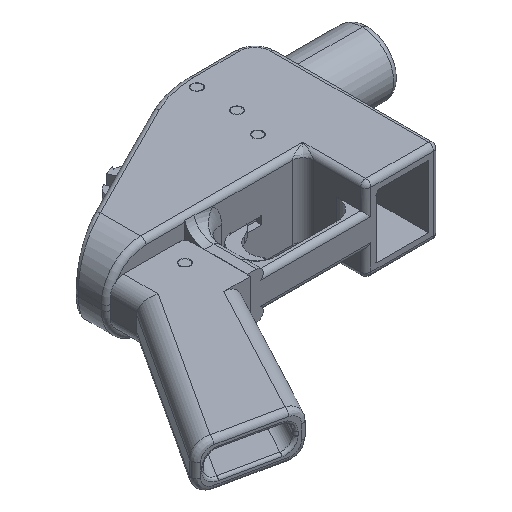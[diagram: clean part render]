
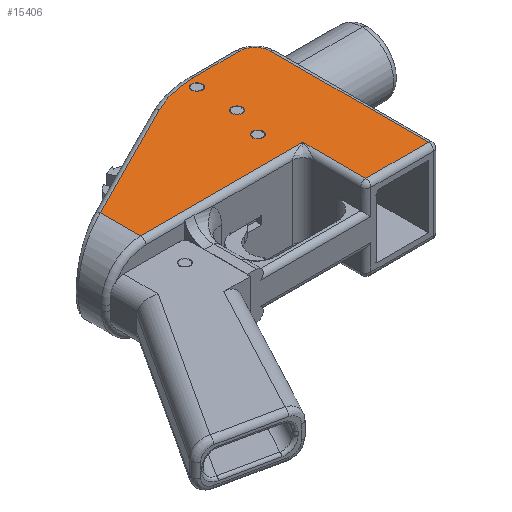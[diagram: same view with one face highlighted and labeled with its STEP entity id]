
A CAD part, isometric view. The second image highlights one B-rep face of the part: STEP entity #15406.
In plain terms, the highlighted planar face has unit normal (0, 0, 1).
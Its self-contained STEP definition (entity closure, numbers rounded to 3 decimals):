
#90 = EDGE_CURVE ( 'NONE', #6622, #9751, #9383, .T. ) ;
#178 = EDGE_CURVE ( 'NONE', #16074, #3045, #4969, .T. ) ;
#243 = VECTOR ( 'NONE', #9661, 1000. ) ;
#358 = DIRECTION ( 'NONE',  ( -0.893, -0.45, 0. ) ) ;
#572 = DIRECTION ( 'NONE',  ( 1., 0., 0. ) ) ;
#606 = DIRECTION ( 'NONE',  ( 1., 0., 0. ) ) ;
#698 = CARTESIAN_POINT ( 'NONE',  ( -33.02, 0., 40.64 ) ) ;
#745 = AXIS2_PLACEMENT_3D ( 'NONE', #16771, #8692, #606 ) ;
#792 = CARTESIAN_POINT ( 'NONE',  ( -32.373, 8.026, 40.64 ) ) ;
#1015 = ORIENTED_EDGE ( 'NONE', *, *, #2822, .F. ) ;
#1487 = PLANE ( 'NONE',  #14224 ) ;
#1628 = CARTESIAN_POINT ( 'NONE',  ( -10.16, 48.666, 40.64 ) ) ;
#1798 = VERTEX_POINT ( 'NONE', #6465 ) ;
#1871 = AXIS2_PLACEMENT_3D ( 'NONE', #6925, #16336, #8287 ) ;
#1890 = FACE_BOUND ( 'NONE', #12005, .T. ) ;
#2166 = DIRECTION ( 'NONE',  ( 1., 0., 0. ) ) ;
#2328 = ORIENTED_EDGE ( 'NONE', *, *, #14817, .T. ) ;
#2641 = EDGE_CURVE ( 'NONE', #2721, #5325, #10907, .T. ) ;
#2650 = CARTESIAN_POINT ( 'NONE',  ( -111.887, 21.996, 40.64 ) ) ;
#2721 = VERTEX_POINT ( 'NONE', #2773 ) ;
#2773 = CARTESIAN_POINT ( 'NONE',  ( -33.02, 32.004, 40.64 ) ) ;
#2795 = ORIENTED_EDGE ( 'NONE', *, *, #5868, .T. ) ;
#2805 = CARTESIAN_POINT ( 'NONE',  ( -32.373, 56.286, 40.64 ) ) ;
#2822 = EDGE_CURVE ( 'NONE', #15205, #1798, #7974, .T. ) ;
#2852 = DIRECTION ( 'NONE',  ( 0., 0., 1. ) ) ;
#2897 = CARTESIAN_POINT ( 'NONE',  ( -33.02, -27.94, 40.64 ) ) ;
#2994 = DIRECTION ( 'NONE',  ( 1., 0., 0. ) ) ;
#3013 = ORIENTED_EDGE ( 'NONE', *, *, #15553, .T. ) ;
#3045 = VERTEX_POINT ( 'NONE', #10293 ) ;
#3214 = ORIENTED_EDGE ( 'NONE', *, *, #6629, .T. ) ;
#3539 = DIRECTION ( 'NONE',  ( 1., 0., 0. ) ) ;
#3587 = CARTESIAN_POINT ( 'NONE',  ( -2.54, -27.94, 40.64 ) ) ;
#3727 = CARTESIAN_POINT ( 'NONE',  ( -35.56, 32.004, 40.64 ) ) ;
#4057 = VECTOR ( 'NONE', #12836, 1000. ) ;
#4969 = LINE ( 'NONE', #8660, #8136 ) ;
#5080 = DIRECTION ( 'NONE',  ( 1., 0., 0. ) ) ;
#5325 = VERTEX_POINT ( 'NONE', #15192 ) ;
#5681 = CARTESIAN_POINT ( 'NONE',  ( -35.56, 51.46, 40.64 ) ) ;
#5856 = VERTEX_POINT ( 'NONE', #2897 ) ;
#5868 = EDGE_CURVE ( 'NONE', #12746, #16471, #7442, .T. ) ;
#6081 = EDGE_CURVE ( 'NONE', #7611, #16074, #7645, .T. ) ;
#6192 = CARTESIAN_POINT ( 'NONE',  ( 0., -27.94, 40.64 ) ) ;
#6370 = ORIENTED_EDGE ( 'NONE', *, *, #14451, .T. ) ;
#6440 = EDGE_LOOP ( 'NONE', ( #9652, #13041, #6370, #2795, #2328, #6658, #3214, #3013, #10388 ) ) ;
#6465 = CARTESIAN_POINT ( 'NONE',  ( -33.02, 51.46, 40.64 ) ) ;
#6622 = VERTEX_POINT ( 'NONE', #11529 ) ;
#6629 = EDGE_CURVE ( 'NONE', #16402, #8328, #9920, .T. ) ;
#6658 = ORIENTED_EDGE ( 'NONE', *, *, #7137, .T. ) ;
#6925 = CARTESIAN_POINT ( 'NONE',  ( -40.64, 16.764, 40.64 ) ) ;
#7032 = ORIENTED_EDGE ( 'NONE', *, *, #90, .F. ) ;
#7036 = DIRECTION ( 'NONE',  ( 1., 0., 0. ) ) ;
#7069 = CARTESIAN_POINT ( 'NONE',  ( -35.56, 51.46, 40.64 ) ) ;
#7137 = EDGE_CURVE ( 'NONE', #11227, #16402, #10328, .T. ) ;
#7325 = EDGE_CURVE ( 'NONE', #3045, #5856, #8636, .T. ) ;
#7442 = LINE ( 'NONE', #8320, #243 ) ;
#7443 = DIRECTION ( 'NONE',  ( 0., -1., 0. ) ) ;
#7601 = CARTESIAN_POINT ( 'NONE',  ( -35.56, 32.004, 40.64 ) ) ;
#7611 = VERTEX_POINT ( 'NONE', #2650 ) ;
#7645 = LINE ( 'NONE', #10128, #4057 ) ;
#7696 = CARTESIAN_POINT ( 'NONE',  ( -38.1, 51.46, 40.64 ) ) ;
#7916 = EDGE_CURVE ( 'NONE', #5325, #2721, #10829, .T. ) ;
#7974 = CIRCLE ( 'NONE', #9037, 2.54 ) ;
#8136 = VECTOR ( 'NONE', #572, 1000. ) ;
#8287 = DIRECTION ( 'NONE',  ( 1., 0., 0. ) ) ;
#8320 = CARTESIAN_POINT ( 'NONE',  ( -2.54, 48.666, 40.64 ) ) ;
#8328 = VERTEX_POINT ( 'NONE', #11096 ) ;
#8422 = DIRECTION ( 'NONE',  ( 1., 0., 0. ) ) ;
#8543 = ORIENTED_EDGE ( 'NONE', *, *, #2641, .F. ) ;
#8633 = FACE_OUTER_BOUND ( 'NONE', #6440, .T. ) ;
#8636 = LINE ( 'NONE', #698, #11377 ) ;
#8660 = CARTESIAN_POINT ( 'NONE',  ( -35.56, 2.54, 40.64 ) ) ;
#8692 = DIRECTION ( 'NONE',  ( 0., 0., 1. ) ) ;
#8703 = CARTESIAN_POINT ( 'NONE',  ( -111.887, 2.54, 40.64 ) ) ;
#8934 = DIRECTION ( 'NONE',  ( 1., 0., 0. ) ) ;
#9037 = AXIS2_PLACEMENT_3D ( 'NONE', #7069, #16488, #8422 ) ;
#9312 = AXIS2_PLACEMENT_3D ( 'NONE', #5681, #15102, #7036 ) ;
#9366 = AXIS2_PLACEMENT_3D ( 'NONE', #792, #10224, #2166 ) ;
#9383 = CIRCLE ( 'NONE', #745, 2.54 ) ;
#9475 = FACE_BOUND ( 'NONE', #13864, .T. ) ;
#9652 = ORIENTED_EDGE ( 'NONE', *, *, #178, .T. ) ;
#9661 = DIRECTION ( 'NONE',  ( 0., 1., 0. ) ) ;
#9751 = VERTEX_POINT ( 'NONE', #15191 ) ;
#9780 = CARTESIAN_POINT ( 'NONE',  ( -110.744, 22.572, 40.64 ) ) ;
#9920 = CIRCLE ( 'NONE', #9366, 48.26 ) ;
#10128 = CARTESIAN_POINT ( 'NONE',  ( -111.887, 0., 40.64 ) ) ;
#10224 = DIRECTION ( 'NONE',  ( 0., 0., 1. ) ) ;
#10280 = AXIS2_PLACEMENT_3D ( 'NONE', #3727, #13144, #5080 ) ;
#10293 = CARTESIAN_POINT ( 'NONE',  ( -33.02, 2.54, 40.64 ) ) ;
#10328 = LINE ( 'NONE', #11142, #17085 ) ;
#10388 = ORIENTED_EDGE ( 'NONE', *, *, #6081, .T. ) ;
#10448 = ORIENTED_EDGE ( 'NONE', *, *, #7916, .F. ) ;
#10829 = CIRCLE ( 'NONE', #15818, 2.54 ) ;
#10907 = CIRCLE ( 'NONE', #10280, 2.54 ) ;
#10910 = CARTESIAN_POINT ( 'NONE',  ( 0., 0., 40.64 ) ) ;
#10949 = LINE ( 'NONE', #9780, #14127 ) ;
#11042 = CARTESIAN_POINT ( 'NONE',  ( -2.54, 48.666, 40.64 ) ) ;
#11055 = DIRECTION ( 'NONE',  ( 0., 0., 1. ) ) ;
#11096 = CARTESIAN_POINT ( 'NONE',  ( -54.092, 51.123, 40.64 ) ) ;
#11142 = CARTESIAN_POINT ( 'NONE',  ( -32.373, 56.286, 40.64 ) ) ;
#11195 = CIRCLE ( 'NONE', #13071, 7.62 ) ;
#11227 = VERTEX_POINT ( 'NONE', #11921 ) ;
#11377 = VECTOR ( 'NONE', #7443, 1000. ) ;
#11463 = EDGE_CURVE ( 'NONE', #1798, #15205, #14997, .T. ) ;
#11529 = CARTESIAN_POINT ( 'NONE',  ( -43.18, 16.764, 40.64 ) ) ;
#11921 = CARTESIAN_POINT ( 'NONE',  ( -10.16, 56.286, 40.64 ) ) ;
#12005 = EDGE_LOOP ( 'NONE', ( #13009, #1015 ) ) ;
#12269 = DIRECTION ( 'NONE',  ( 1., 0., 0. ) ) ;
#12476 = DIRECTION ( 'NONE',  ( -1., 0., 0. ) ) ;
#12746 = VERTEX_POINT ( 'NONE', #3587 ) ;
#12836 = DIRECTION ( 'NONE',  ( 0., -1., 0. ) ) ;
#13009 = ORIENTED_EDGE ( 'NONE', *, *, #11463, .F. ) ;
#13011 = EDGE_CURVE ( 'NONE', #9751, #6622, #15986, .T. ) ;
#13041 = ORIENTED_EDGE ( 'NONE', *, *, #7325, .T. ) ;
#13071 = AXIS2_PLACEMENT_3D ( 'NONE', #1628, #11055, #2994 ) ;
#13144 = DIRECTION ( 'NONE',  ( 0., 0., 1. ) ) ;
#13616 = VECTOR ( 'NONE', #3539, 1000. ) ;
#13864 = EDGE_LOOP ( 'NONE', ( #15035, #7032 ) ) ;
#14127 = VECTOR ( 'NONE', #358, 1000. ) ;
#14224 = AXIS2_PLACEMENT_3D ( 'NONE', #10910, #2852, #12269 ) ;
#14404 = EDGE_LOOP ( 'NONE', ( #8543, #10448 ) ) ;
#14451 = EDGE_CURVE ( 'NONE', #5856, #12746, #14573, .T. ) ;
#14573 = LINE ( 'NONE', #6192, #13616 ) ;
#14817 = EDGE_CURVE ( 'NONE', #16471, #11227, #11195, .T. ) ;
#14997 = CIRCLE ( 'NONE', #9312, 2.54 ) ;
#15035 = ORIENTED_EDGE ( 'NONE', *, *, #13011, .F. ) ;
#15102 = DIRECTION ( 'NONE',  ( 0., 0., 1. ) ) ;
#15191 = CARTESIAN_POINT ( 'NONE',  ( -38.1, 16.764, 40.64 ) ) ;
#15192 = CARTESIAN_POINT ( 'NONE',  ( -38.1, 32.004, 40.64 ) ) ;
#15205 = VERTEX_POINT ( 'NONE', #7696 ) ;
#15406 = ADVANCED_FACE ( 'NONE', ( #9475, #15807, #1890, #8633 ), #1487, .T. ) ;
#15553 = EDGE_CURVE ( 'NONE', #8328, #7611, #10949, .T. ) ;
#15807 = FACE_BOUND ( 'NONE', #14404, .T. ) ;
#15818 = AXIS2_PLACEMENT_3D ( 'NONE', #7601, #17003, #8934 ) ;
#15986 = CIRCLE ( 'NONE', #1871, 2.54 ) ;
#16074 = VERTEX_POINT ( 'NONE', #8703 ) ;
#16336 = DIRECTION ( 'NONE',  ( 0., 0., 1. ) ) ;
#16402 = VERTEX_POINT ( 'NONE', #2805 ) ;
#16471 = VERTEX_POINT ( 'NONE', #11042 ) ;
#16488 = DIRECTION ( 'NONE',  ( 0., 0., 1. ) ) ;
#16771 = CARTESIAN_POINT ( 'NONE',  ( -40.64, 16.764, 40.64 ) ) ;
#17003 = DIRECTION ( 'NONE',  ( 0., 0., 1. ) ) ;
#17085 = VECTOR ( 'NONE', #12476, 1000. ) ;
